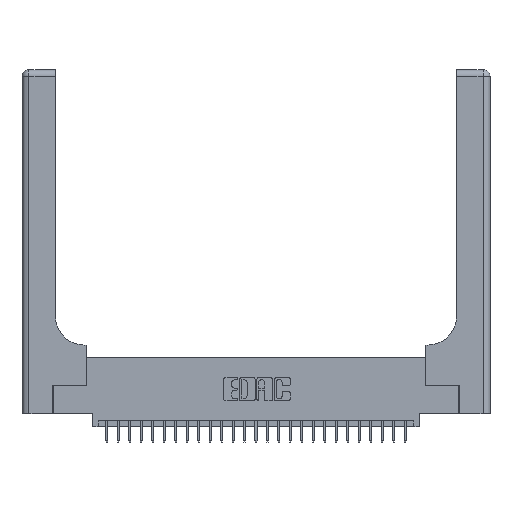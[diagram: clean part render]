
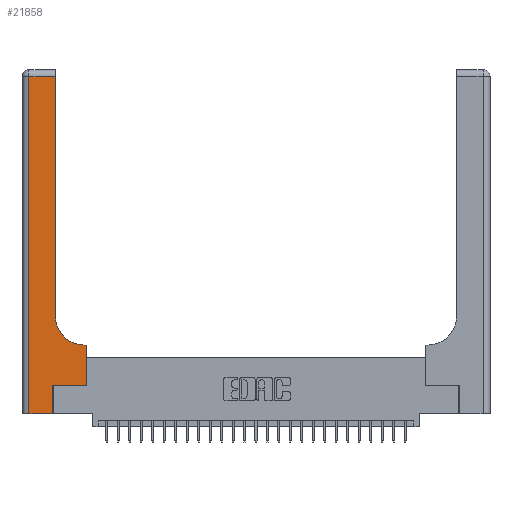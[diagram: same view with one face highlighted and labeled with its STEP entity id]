
A CAD part, top view. The second image highlights one B-rep face of the part: STEP entity #21858.
In plain terms, the highlighted planar face has unit normal (0, 0, 1).
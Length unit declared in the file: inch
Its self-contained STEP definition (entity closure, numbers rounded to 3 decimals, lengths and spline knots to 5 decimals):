
#146 = CARTESIAN_POINT ( 'NONE',  ( 0.5585, 0.25, 0.37 ) ) ;
#811 = VERTEX_POINT ( 'NONE', #22924 ) ;
#1065 = ORIENTED_EDGE ( 'NONE', *, *, #26236, .T. ) ;
#1066 = CARTESIAN_POINT ( 'NONE',  ( 0.2915, 0.6, 0.37 ) ) ;
#1594 = CARTESIAN_POINT ( 'NONE',  ( 0., 3., 0.37 ) ) ;
#1848 = VECTOR ( 'NONE', #27288, 39.37008 ) ;
#1883 = PLANE ( 'NONE',  #22105 ) ;
#1897 = LINE ( 'NONE', #6261, #25021 ) ;
#1966 = CARTESIAN_POINT ( 'NONE',  ( 0.2915, 2.94, 0.37 ) ) ;
#2002 = CARTESIAN_POINT ( 'NONE',  ( 0.269, 0.25, 0.37 ) ) ;
#3234 = CARTESIAN_POINT ( 'NONE',  ( 0.269, 0., 0.37 ) ) ;
#3808 = DIRECTION ( 'NONE',  ( 0., 0., -1. ) ) ;
#3905 = VECTOR ( 'NONE', #16011, 39.37008 ) ;
#4477 = CARTESIAN_POINT ( 'NONE',  ( 0., 0., 0.37 ) ) ;
#4539 = ORIENTED_EDGE ( 'NONE', *, *, #20590, .T. ) ;
#5584 = VERTEX_POINT ( 'NONE', #3234 ) ;
#6261 = CARTESIAN_POINT ( 'NONE',  ( 0.5585, 0.25, 0.37 ) ) ;
#6297 = CARTESIAN_POINT ( 'NONE',  ( 0.5585, 0.6, 0.37 ) ) ;
#6467 = VECTOR ( 'NONE', #9508, 39.37008 ) ;
#8287 = DIRECTION ( 'NONE',  ( 0., 1., 0. ) ) ;
#8329 = ORIENTED_EDGE ( 'NONE', *, *, #25528, .T. ) ;
#8961 = VERTEX_POINT ( 'NONE', #26832 ) ;
#9098 = LINE ( 'NONE', #18082, #19021 ) ;
#9447 = DIRECTION ( 'NONE',  ( 0., 1., 0. ) ) ;
#9508 = DIRECTION ( 'NONE',  ( 0., -1., 0. ) ) ;
#9534 = AXIS2_PLACEMENT_3D ( 'NONE', #28266, #3808, #10204 ) ;
#9778 = ORIENTED_EDGE ( 'NONE', *, *, #27258, .T. ) ;
#9940 = VECTOR ( 'NONE', #15374, 39.37008 ) ;
#10066 = VERTEX_POINT ( 'NONE', #27333 ) ;
#10204 = DIRECTION ( 'NONE',  ( 1., 0., 0. ) ) ;
#10386 = VERTEX_POINT ( 'NONE', #1966 ) ;
#10662 = ORIENTED_EDGE ( 'NONE', *, *, #18789, .T. ) ;
#11072 = EDGE_CURVE ( 'NONE', #25219, #11944, #1897, .T. ) ;
#11782 = ORIENTED_EDGE ( 'NONE', *, *, #15012, .T. ) ;
#11815 = ORIENTED_EDGE ( 'NONE', *, *, #11072, .T. ) ;
#11944 = VERTEX_POINT ( 'NONE', #6297 ) ;
#12100 = ORIENTED_EDGE ( 'NONE', *, *, #22548, .T. ) ;
#15012 = EDGE_CURVE ( 'NONE', #811, #10386, #18449, .T. ) ;
#15374 = DIRECTION ( 'NONE',  ( 1., 0., 0. ) ) ;
#15660 = EDGE_CURVE ( 'NONE', #10066, #5584, #16836, .T. ) ;
#15703 = EDGE_LOOP ( 'NONE', ( #11782, #9778, #8329, #25971, #4539, #12100, #11815, #1065, #10662 ) ) ;
#16011 = DIRECTION ( 'NONE',  ( 0., 1., 0. ) ) ;
#16296 = VERTEX_POINT ( 'NONE', #20523 ) ;
#16406 = CARTESIAN_POINT ( 'NONE',  ( 0.269, 0., 0.37 ) ) ;
#16836 = LINE ( 'NONE', #4477, #9940 ) ;
#16953 = DIRECTION ( 'NONE',  ( 1., 0., 0. ) ) ;
#17265 = DIRECTION ( 'NONE',  ( -1., 0., 0. ) ) ;
#18056 = CARTESIAN_POINT ( 'NONE',  ( 0.06, 3., 0.37 ) ) ;
#18082 = CARTESIAN_POINT ( 'NONE',  ( 0., 2.94, 0.37 ) ) ;
#18449 = LINE ( 'NONE', #27137, #3905 ) ;
#18789 = EDGE_CURVE ( 'NONE', #21638, #811, #20161, .T. ) ;
#19021 = VECTOR ( 'NONE', #19690, 39.37008 ) ;
#19690 = DIRECTION ( 'NONE',  ( -1., 0., 0. ) ) ;
#20161 = CIRCLE ( 'NONE', #9534, 0.25 ) ;
#20523 = CARTESIAN_POINT ( 'NONE',  ( 0.06, 2.94, 0.37 ) ) ;
#20590 = EDGE_CURVE ( 'NONE', #5584, #8961, #24945, .T. ) ;
#20732 = CARTESIAN_POINT ( 'NONE',  ( 0.5415, 0.6, 0.37 ) ) ;
#21638 = VERTEX_POINT ( 'NONE', #20732 ) ;
#21694 = LINE ( 'NONE', #2002, #23491 ) ;
#21858 = ADVANCED_FACE ( 'NONE', ( #23916 ), #1883, .F. ) ;
#22105 = AXIS2_PLACEMENT_3D ( 'NONE', #1594, #25798, #17265 ) ;
#22548 = EDGE_CURVE ( 'NONE', #8961, #25219, #21694, .T. ) ;
#22924 = CARTESIAN_POINT ( 'NONE',  ( 0.2915, 0.85, 0.37 ) ) ;
#23387 = LINE ( 'NONE', #1066, #1848 ) ;
#23478 = VECTOR ( 'NONE', #9447, 39.37008 ) ;
#23491 = VECTOR ( 'NONE', #16953, 39.37008 ) ;
#23916 = FACE_OUTER_BOUND ( 'NONE', #15703, .T. ) ;
#24945 = LINE ( 'NONE', #16406, #23478 ) ;
#25021 = VECTOR ( 'NONE', #8287, 39.37008 ) ;
#25219 = VERTEX_POINT ( 'NONE', #146 ) ;
#25528 = EDGE_CURVE ( 'NONE', #16296, #10066, #26593, .T. ) ;
#25798 = DIRECTION ( 'NONE',  ( 0., 0., -1. ) ) ;
#25971 = ORIENTED_EDGE ( 'NONE', *, *, #15660, .T. ) ;
#26236 = EDGE_CURVE ( 'NONE', #11944, #21638, #23387, .T. ) ;
#26593 = LINE ( 'NONE', #18056, #6467 ) ;
#26832 = CARTESIAN_POINT ( 'NONE',  ( 0.269, 0.25, 0.37 ) ) ;
#27137 = CARTESIAN_POINT ( 'NONE',  ( 0.2915, 3., 0.37 ) ) ;
#27258 = EDGE_CURVE ( 'NONE', #10386, #16296, #9098, .T. ) ;
#27288 = DIRECTION ( 'NONE',  ( -1., 0., 0. ) ) ;
#27333 = CARTESIAN_POINT ( 'NONE',  ( 0.06, 0., 0.37 ) ) ;
#28266 = CARTESIAN_POINT ( 'NONE',  ( 0.5415, 0.85, 0.37 ) ) ;
